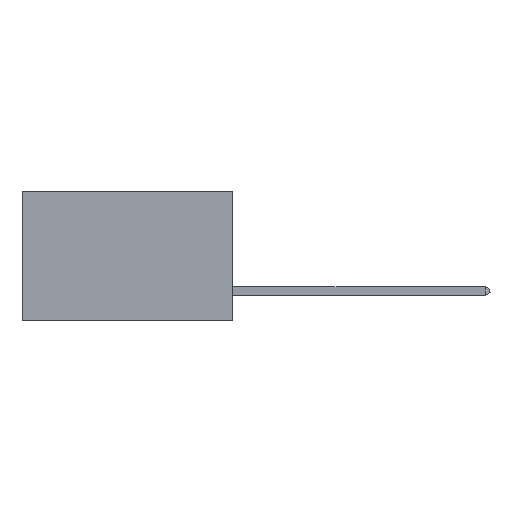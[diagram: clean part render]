
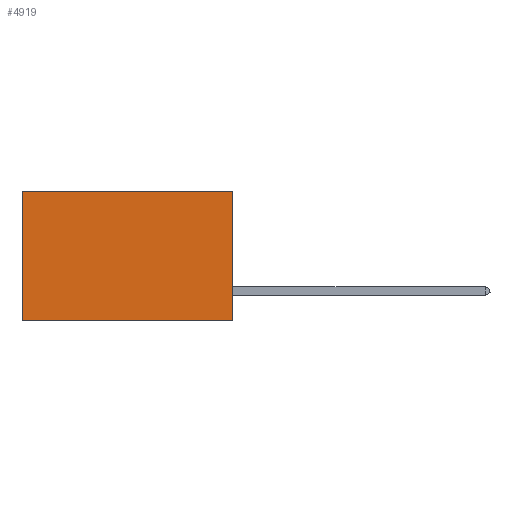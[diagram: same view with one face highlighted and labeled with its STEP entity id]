
A CAD part, left-side view. The second image highlights one B-rep face of the part: STEP entity #4919.
In plain terms, the highlighted planar face has unit normal (-1, 0, 0).
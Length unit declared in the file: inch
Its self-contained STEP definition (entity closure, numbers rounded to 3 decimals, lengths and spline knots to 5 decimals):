
#381 = DIRECTION ( 'NONE',  ( 0., 0., -1. ) ) ;
#409 = CARTESIAN_POINT ( 'NONE',  ( 0.2875, 0., -0.37 ) ) ;
#412 = PLANE ( 'NONE',  #8035 ) ;
#910 = DIRECTION ( 'NONE',  ( 0., 0., -1. ) ) ;
#1477 = VECTOR ( 'NONE', #2305, 39.37008 ) ;
#1624 = LINE ( 'NONE', #5922, #1477 ) ;
#2198 = DIRECTION ( 'NONE',  ( 0., 1., 0. ) ) ;
#2305 = DIRECTION ( 'NONE',  ( 0., 0., -1. ) ) ;
#2695 = VECTOR ( 'NONE', #4962, 39.37008 ) ;
#2820 = EDGE_LOOP ( 'NONE', ( #7796, #2939, #4672, #11990 ) ) ;
#2843 = VECTOR ( 'NONE', #2198, 39.37008 ) ;
#2939 = ORIENTED_EDGE ( 'NONE', *, *, #8425, .F. ) ;
#3259 = CARTESIAN_POINT ( 'NONE',  ( 0.2875, 0., -0.37 ) ) ;
#3729 = LINE ( 'NONE', #11312, #10846 ) ;
#4042 = LINE ( 'NONE', #409, #2843 ) ;
#4046 = VERTEX_POINT ( 'NONE', #3259 ) ;
#4239 = VERTEX_POINT ( 'NONE', #9017 ) ;
#4672 = ORIENTED_EDGE ( 'NONE', *, *, #4997, .F. ) ;
#4919 = ADVANCED_FACE ( 'NONE', ( #9306 ), #412, .F. ) ;
#4962 = DIRECTION ( 'NONE',  ( 0., 1., 0. ) ) ;
#4997 = EDGE_CURVE ( 'NONE', #4239, #4046, #1624, .T. ) ;
#5922 = CARTESIAN_POINT ( 'NONE',  ( 0.2875, 0., 0. ) ) ;
#5999 = CARTESIAN_POINT ( 'NONE',  ( 0.2875, 0., 0. ) ) ;
#6074 = LINE ( 'NONE', #10510, #2695 ) ;
#6174 = CARTESIAN_POINT ( 'NONE',  ( 0.2875, 0.6, 0. ) ) ;
#7796 = ORIENTED_EDGE ( 'NONE', *, *, #8817, .T. ) ;
#7857 = DIRECTION ( 'NONE',  ( 1., 0., 0. ) ) ;
#8035 = AXIS2_PLACEMENT_3D ( 'NONE', #5999, #7857, #381 ) ;
#8425 = EDGE_CURVE ( 'NONE', #4046, #11368, #4042, .T. ) ;
#8469 = CARTESIAN_POINT ( 'NONE',  ( 0.2875, 0.6, -0.37 ) ) ;
#8732 = EDGE_CURVE ( 'NONE', #4239, #10325, #6074, .T. ) ;
#8817 = EDGE_CURVE ( 'NONE', #10325, #11368, #3729, .T. ) ;
#9017 = CARTESIAN_POINT ( 'NONE',  ( 0.2875, 0., 0. ) ) ;
#9306 = FACE_OUTER_BOUND ( 'NONE', #2820, .T. ) ;
#10325 = VERTEX_POINT ( 'NONE', #6174 ) ;
#10510 = CARTESIAN_POINT ( 'NONE',  ( 0.2875, 0., 0. ) ) ;
#10846 = VECTOR ( 'NONE', #910, 39.37008 ) ;
#11312 = CARTESIAN_POINT ( 'NONE',  ( 0.2875, 0.6, 0. ) ) ;
#11368 = VERTEX_POINT ( 'NONE', #8469 ) ;
#11990 = ORIENTED_EDGE ( 'NONE', *, *, #8732, .T. ) ;
